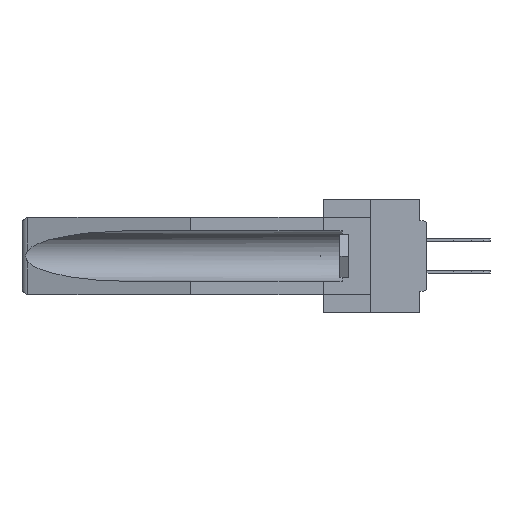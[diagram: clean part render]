
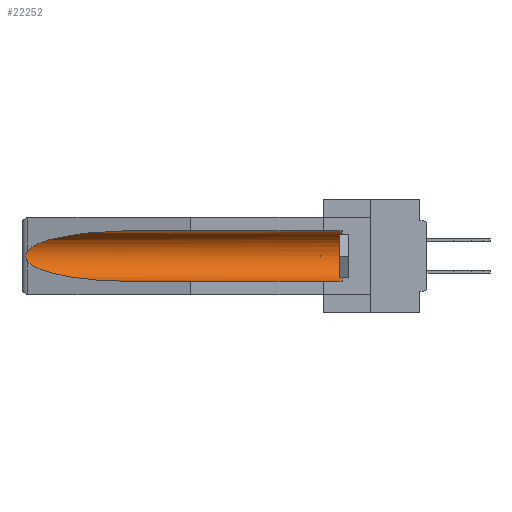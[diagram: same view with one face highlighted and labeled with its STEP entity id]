
A CAD part, left-side view. The second image highlights one B-rep face of the part: STEP entity #22252.
In plain terms, the highlighted cylindrical face has radius 2.857 mm (diameter 5.715 mm), a partial arc.
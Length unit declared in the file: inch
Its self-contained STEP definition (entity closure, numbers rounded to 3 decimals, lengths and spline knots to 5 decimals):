
#6 = VECTOR ( 'NONE', #33658, 39.37008 ) ;
#378 =( BOUNDED_CURVE ( )  B_SPLINE_CURVE ( 3, ( #8253, #12123, #12289, #42082 ),
 .UNSPECIFIED., .F., .T. ) 
 B_SPLINE_CURVE_WITH_KNOTS ( ( 4, 4 ),
 ( 4.71239, 6.08839 ),
 .UNSPECIFIED. ) 
 CURVE ( )  GEOMETRIC_REPRESENTATION_ITEM ( )  RATIONAL_B_SPLINE_CURVE ( ( 1., 0.848, 0.848, 1. ) ) 
 REPRESENTATION_ITEM ( '' )  );
#447 = EDGE_CURVE ( 'NONE', #38803, #28397, #378, .T. ) ;
#637 = CARTESIAN_POINT ( 'NONE',  ( 0.26597, 1.5296, -0.19026 ) ) ;
#1096 = EDGE_LOOP ( 'NONE', ( #16498, #3419, #37120, #25383, #28202, #12089 ) ) ;
#1159 = DIRECTION ( 'NONE',  ( 0., -1., 0. ) ) ;
#3174 = CARTESIAN_POINT ( 'NONE',  ( 0.155, 1.07973, -0.284 ) ) ;
#3419 = ORIENTED_EDGE ( 'NONE', *, *, #8941, .T. ) ;
#4244 = LINE ( 'NONE', #27808, #28515 ) ;
#5440 = CARTESIAN_POINT ( 'NONE',  ( 0.26537, 1.52718, -0.19328 ) ) ;
#7414 = AXIS2_PLACEMENT_3D ( 'NONE', #9595, #42805, #28205 ) ;
#8253 = CARTESIAN_POINT ( 'NONE',  ( 0.155, 1.07973, -0.059 ) ) ;
#8538 = DIRECTION ( 'NONE',  ( 0., 0., 1. ) ) ;
#8941 = EDGE_CURVE ( 'NONE', #28397, #29515, #20235, .T. ) ;
#9595 = CARTESIAN_POINT ( 'NONE',  ( 0.155, -0.30754, -0.1715 ) ) ;
#9803 = LINE ( 'NONE', #43604, #6 ) ;
#12089 = ORIENTED_EDGE ( 'NONE', *, *, #39561, .T. ) ;
#12123 = CARTESIAN_POINT ( 'NONE',  ( 0.21114, 1.30732, -0.059 ) ) ;
#12289 = CARTESIAN_POINT ( 'NONE',  ( 0.25451, 1.48313, -0.09465 ) ) ;
#15310 = CARTESIAN_POINT ( 'NONE',  ( 0.2675, 1.53308, -0.17534 ) ) ;
#15465 = CARTESIAN_POINT ( 'NONE',  ( 0.26537, 1.52718, -0.19328 ) ) ;
#16498 = ORIENTED_EDGE ( 'NONE', *, *, #447, .T. ) ;
#17409 = CARTESIAN_POINT ( 'NONE',  ( 0.26537, 1.52718, -0.14972 ) ) ;
#19375 = CARTESIAN_POINT ( 'NONE',  ( 0.26537, 1.52718, -0.14972 ) ) ;
#20134 = CARTESIAN_POINT ( 'NONE',  ( 0.155, 1.07973, -0.284 ) ) ;
#20235 = B_SPLINE_CURVE_WITH_KNOTS ( 'NONE', 3,
 ( #19375, #41539, #44935, #37491, #26475, #15310, #41221, #45430, #637, #15465 ),
 .UNSPECIFIED., .F., .F.,
 ( 4, 2, 2, 2, 4 ),
 ( 0., 0.00029, 0.00058, 0.00087, 0.00117 ),
 .UNSPECIFIED. ) ;
#22252 = ADVANCED_FACE ( 'NONE', ( #30742 ), #46994, .F. ) ;
#24646 = VERTEX_POINT ( 'NONE', #31094 ) ;
#25383 = ORIENTED_EDGE ( 'NONE', *, *, #47647, .F. ) ;
#26475 = CARTESIAN_POINT ( 'NONE',  ( 0.2675, 1.53308, -0.16763 ) ) ;
#27808 = CARTESIAN_POINT ( 'NONE',  ( 0.155, -0.30754, -0.059 ) ) ;
#28202 = ORIENTED_EDGE ( 'NONE', *, *, #28717, .T. ) ;
#28205 = DIRECTION ( 'NONE',  ( 0., 0., 1. ) ) ;
#28397 = VERTEX_POINT ( 'NONE', #17409 ) ;
#28515 = VECTOR ( 'NONE', #42879, 39.37008 ) ;
#28717 = EDGE_CURVE ( 'NONE', #24646, #43408, #47628, .T. ) ;
#29258 = VERTEX_POINT ( 'NONE', #3174 ) ;
#29515 = VERTEX_POINT ( 'NONE', #44580 ) ;
#30723 = CARTESIAN_POINT ( 'NONE',  ( 0.155, 0.126, -0.059 ) ) ;
#30742 = FACE_OUTER_BOUND ( 'NONE', #1096, .T. ) ;
#31094 = CARTESIAN_POINT ( 'NONE',  ( 0.155, 0.126, -0.284 ) ) ;
#32033 = EDGE_CURVE ( 'NONE', #29515, #29258, #43394, .T. ) ;
#33658 = DIRECTION ( 'NONE',  ( 0., 1., 0. ) ) ;
#34821 = CARTESIAN_POINT ( 'NONE',  ( 0.21114, 1.30732, -0.284 ) ) ;
#37120 = ORIENTED_EDGE ( 'NONE', *, *, #32033, .T. ) ;
#37491 = CARTESIAN_POINT ( 'NONE',  ( 0.2673, 1.5327, -0.16383 ) ) ;
#37740 = CARTESIAN_POINT ( 'NONE',  ( 0.155, 1.07973, -0.059 ) ) ;
#38175 = CARTESIAN_POINT ( 'NONE',  ( 0.155, 0.126, -0.1715 ) ) ;
#38803 = VERTEX_POINT ( 'NONE', #37740 ) ;
#39561 = EDGE_CURVE ( 'NONE', #43408, #38803, #4244, .T. ) ;
#41221 = CARTESIAN_POINT ( 'NONE',  ( 0.2673, 1.53269, -0.17917 ) ) ;
#41539 = CARTESIAN_POINT ( 'NONE',  ( 0.26597, 1.52961, -0.15275 ) ) ;
#42082 = CARTESIAN_POINT ( 'NONE',  ( 0.26537, 1.52718, -0.14972 ) ) ;
#42484 = CARTESIAN_POINT ( 'NONE',  ( 0.25451, 1.48313, -0.24835 ) ) ;
#42805 = DIRECTION ( 'NONE',  ( 0., 1., 0. ) ) ;
#42879 = DIRECTION ( 'NONE',  ( 0., 1., 0. ) ) ;
#43394 =( BOUNDED_CURVE ( )  B_SPLINE_CURVE ( 3, ( #5440, #42484, #34821, #20134 ),
 .UNSPECIFIED., .F., .F. ) 
 B_SPLINE_CURVE_WITH_KNOTS ( ( 4, 4 ),
 ( 0.1948, 1.5708 ),
 .UNSPECIFIED. ) 
 CURVE ( )  GEOMETRIC_REPRESENTATION_ITEM ( )  RATIONAL_B_SPLINE_CURVE ( ( 1., 0.848, 0.848, 1. ) ) 
 REPRESENTATION_ITEM ( '' )  );
#43408 = VERTEX_POINT ( 'NONE', #30723 ) ;
#43604 = CARTESIAN_POINT ( 'NONE',  ( 0.155, -0.30754, -0.284 ) ) ;
#44580 = CARTESIAN_POINT ( 'NONE',  ( 0.26537, 1.52718, -0.19328 ) ) ;
#44935 = CARTESIAN_POINT ( 'NONE',  ( 0.26654, 1.53092, -0.15636 ) ) ;
#45188 = AXIS2_PLACEMENT_3D ( 'NONE', #38175, #1159, #8538 ) ;
#45430 = CARTESIAN_POINT ( 'NONE',  ( 0.26655, 1.53094, -0.18657 ) ) ;
#46994 = CYLINDRICAL_SURFACE ( 'NONE', #7414, 0.1125 ) ;
#47628 = CIRCLE ( 'NONE', #45188, 0.1125 ) ;
#47647 = EDGE_CURVE ( 'NONE', #24646, #29258, #9803, .T. ) ;
